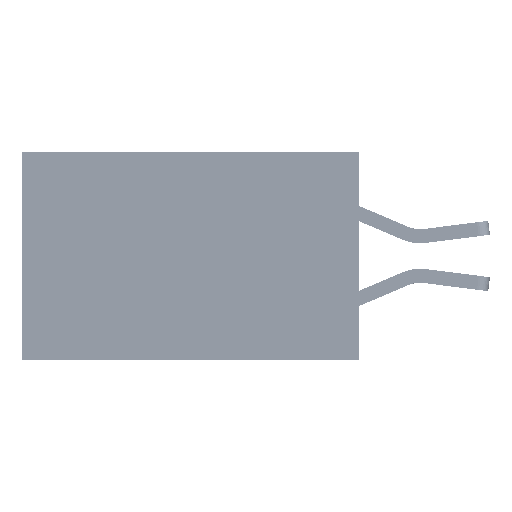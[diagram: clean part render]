
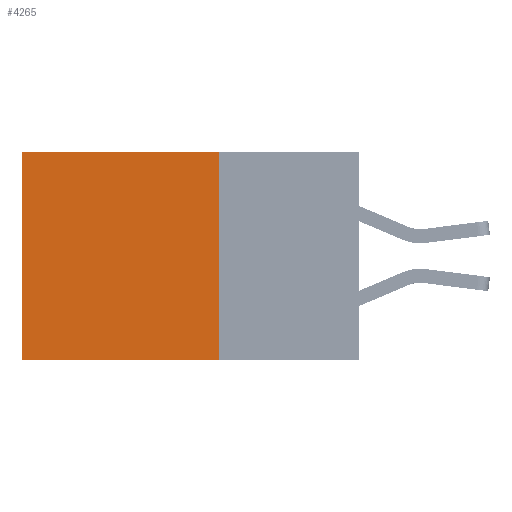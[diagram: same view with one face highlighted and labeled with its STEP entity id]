
A CAD part, left-side view. The second image highlights one B-rep face of the part: STEP entity #4265.
In plain terms, the highlighted planar face has unit normal (-1, 0, 0).
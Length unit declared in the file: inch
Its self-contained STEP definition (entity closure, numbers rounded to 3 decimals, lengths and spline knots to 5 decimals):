
#110 = DIRECTION ( 'NONE',  ( 1., 0., 0. ) ) ;
#366 = CARTESIAN_POINT ( 'NONE',  ( 0.2875, 0.25, 0. ) ) ;
#3181 = LINE ( 'NONE', #44656, #48606 ) ;
#3184 = VECTOR ( 'NONE', #31367, 39.37008 ) ;
#3450 = ORIENTED_EDGE ( 'NONE', *, *, #14066, .T. ) ;
#4265 = ADVANCED_FACE ( 'NONE', ( #40299 ), #47928, .F. ) ;
#4694 = AXIS2_PLACEMENT_3D ( 'NONE', #16287, #110, #44107 ) ;
#7012 = VERTEX_POINT ( 'NONE', #28700 ) ;
#13131 = VERTEX_POINT ( 'NONE', #23084 ) ;
#13252 = EDGE_CURVE ( 'NONE', #13131, #7012, #45502, .T. ) ;
#14066 = EDGE_CURVE ( 'NONE', #47100, #13131, #46760, .T. ) ;
#16287 = CARTESIAN_POINT ( 'NONE',  ( 0.2875, 0.25, 0. ) ) ;
#18013 = EDGE_CURVE ( 'NONE', #47100, #34490, #37567, .T. ) ;
#23084 = CARTESIAN_POINT ( 'NONE',  ( 0.2875, 0.6, 0. ) ) ;
#26975 = VECTOR ( 'NONE', #48368, 39.37008 ) ;
#27093 = CARTESIAN_POINT ( 'NONE',  ( 0.2875, 0.25, 0. ) ) ;
#27675 = ORIENTED_EDGE ( 'NONE', *, *, #37286, .F. ) ;
#28349 = ORIENTED_EDGE ( 'NONE', *, *, #13252, .T. ) ;
#28700 = CARTESIAN_POINT ( 'NONE',  ( 0.2875, 0.6, -0.37 ) ) ;
#31367 = DIRECTION ( 'NONE',  ( 0., 0., -1. ) ) ;
#33663 = VECTOR ( 'NONE', #44020, 39.37008 ) ;
#34412 = ORIENTED_EDGE ( 'NONE', *, *, #18013, .F. ) ;
#34490 = VERTEX_POINT ( 'NONE', #34963 ) ;
#34963 = CARTESIAN_POINT ( 'NONE',  ( 0.2875, 0.25, -0.37 ) ) ;
#37286 = EDGE_CURVE ( 'NONE', #34490, #7012, #3181, .T. ) ;
#37567 = LINE ( 'NONE', #40351, #26975 ) ;
#40299 = FACE_OUTER_BOUND ( 'NONE', #49378, .T. ) ;
#40351 = CARTESIAN_POINT ( 'NONE',  ( 0.2875, 0.25, 0. ) ) ;
#44020 = DIRECTION ( 'NONE',  ( 0., 1., 0. ) ) ;
#44107 = DIRECTION ( 'NONE',  ( 0., 0., -1. ) ) ;
#44656 = CARTESIAN_POINT ( 'NONE',  ( 0.2875, 0.25, -0.37 ) ) ;
#45502 = LINE ( 'NONE', #46534, #3184 ) ;
#46534 = CARTESIAN_POINT ( 'NONE',  ( 0.2875, 0.6, 0. ) ) ;
#46760 = LINE ( 'NONE', #366, #33663 ) ;
#47100 = VERTEX_POINT ( 'NONE', #27093 ) ;
#47928 = PLANE ( 'NONE',  #4694 ) ;
#48368 = DIRECTION ( 'NONE',  ( 0., 0., -1. ) ) ;
#48606 = VECTOR ( 'NONE', #48649, 39.37008 ) ;
#48649 = DIRECTION ( 'NONE',  ( 0., 1., 0. ) ) ;
#49378 = EDGE_LOOP ( 'NONE', ( #28349, #27675, #34412, #3450 ) ) ;
